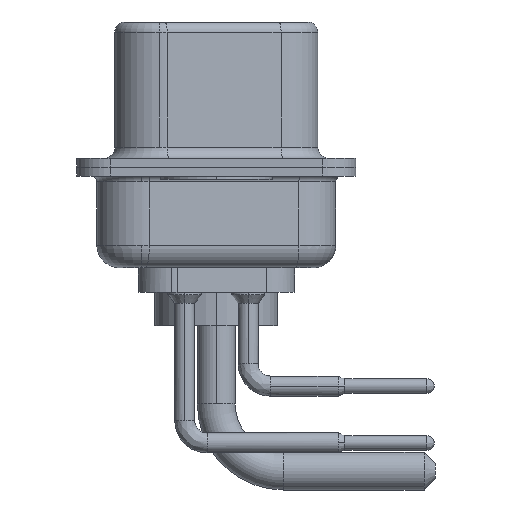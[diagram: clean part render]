
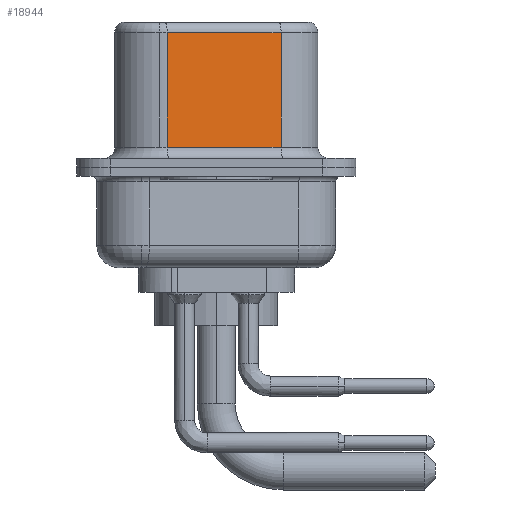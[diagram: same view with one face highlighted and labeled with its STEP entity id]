
A CAD part, left-side view. The second image highlights one B-rep face of the part: STEP entity #18944.
In plain terms, the highlighted planar face has unit normal (-0.985, -0.174, 0).
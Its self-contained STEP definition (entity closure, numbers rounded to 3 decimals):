
#218 = DIRECTION ( 'NONE',  ( 0., 0., -1. ) ) ;
#372 = CARTESIAN_POINT ( 'NONE',  ( 3.68, 2.203, 0.9 ) ) ;
#996 = VERTEX_POINT ( 'NONE', #372 ) ;
#1106 = FACE_OUTER_BOUND ( 'NONE', #1775, .T. ) ;
#1775 = EDGE_LOOP ( 'NONE', ( #23310, #19454, #22395, #9063 ) ) ;
#4502 = DIRECTION ( 'NONE',  ( 0.174, -0.985, 0. ) ) ;
#4862 = AXIS2_PLACEMENT_3D ( 'NONE', #8558, #17315, #23047 ) ;
#5116 = EDGE_CURVE ( 'NONE', #996, #23248, #8185, .T. ) ;
#5137 = LINE ( 'NONE', #10969, #8118 ) ;
#6357 = VERTEX_POINT ( 'NONE', #8559 ) ;
#6544 = EDGE_CURVE ( 'NONE', #6357, #15785, #5137, .T. ) ;
#6875 = CARTESIAN_POINT ( 'NONE',  ( 4.58, -2.897, 0.9 ) ) ;
#7106 = CARTESIAN_POINT ( 'NONE',  ( 4.58, -2.897, 6.52 ) ) ;
#7859 = VECTOR ( 'NONE', #218, 1000. ) ;
#8118 = VECTOR ( 'NONE', #8686, 1000. ) ;
#8185 = LINE ( 'NONE', #13777, #10879 ) ;
#8558 = CARTESIAN_POINT ( 'NONE',  ( 4.58, -2.897, 6.52 ) ) ;
#8559 = CARTESIAN_POINT ( 'NONE',  ( 4.58, -2.897, 6.02 ) ) ;
#8686 = DIRECTION ( 'NONE',  ( -0.174, 0.985, 0. ) ) ;
#9063 = ORIENTED_EDGE ( 'NONE', *, *, #5116, .T. ) ;
#10879 = VECTOR ( 'NONE', #4502, 1000. ) ;
#10969 = CARTESIAN_POINT ( 'NONE',  ( 4.58, -2.897, 6.02 ) ) ;
#12248 = EDGE_CURVE ( 'NONE', #6357, #23248, #22759, .T. ) ;
#13683 = CARTESIAN_POINT ( 'NONE',  ( 3.68, 2.203, 6.02 ) ) ;
#13777 = CARTESIAN_POINT ( 'NONE',  ( 4.58, -2.897, 0.9 ) ) ;
#14497 = DIRECTION ( 'NONE',  ( 0., 0., -1. ) ) ;
#15785 = VERTEX_POINT ( 'NONE', #13683 ) ;
#17315 = DIRECTION ( 'NONE',  ( 0.985, 0.174, 0. ) ) ;
#18139 = LINE ( 'NONE', #21932, #18586 ) ;
#18586 = VECTOR ( 'NONE', #14497, 1000. ) ;
#18944 = ADVANCED_FACE ( 'NONE', ( #1106 ), #21096, .F. ) ;
#19454 = ORIENTED_EDGE ( 'NONE', *, *, #6544, .T. ) ;
#21096 = PLANE ( 'NONE',  #4862 ) ;
#21932 = CARTESIAN_POINT ( 'NONE',  ( 3.68, 2.203, 6.52 ) ) ;
#22395 = ORIENTED_EDGE ( 'NONE', *, *, #22902, .T. ) ;
#22759 = LINE ( 'NONE', #7106, #7859 ) ;
#22902 = EDGE_CURVE ( 'NONE', #15785, #996, #18139, .T. ) ;
#23047 = DIRECTION ( 'NONE',  ( -0.174, 0.985, 0. ) ) ;
#23248 = VERTEX_POINT ( 'NONE', #6875 ) ;
#23310 = ORIENTED_EDGE ( 'NONE', *, *, #12248, .F. ) ;
